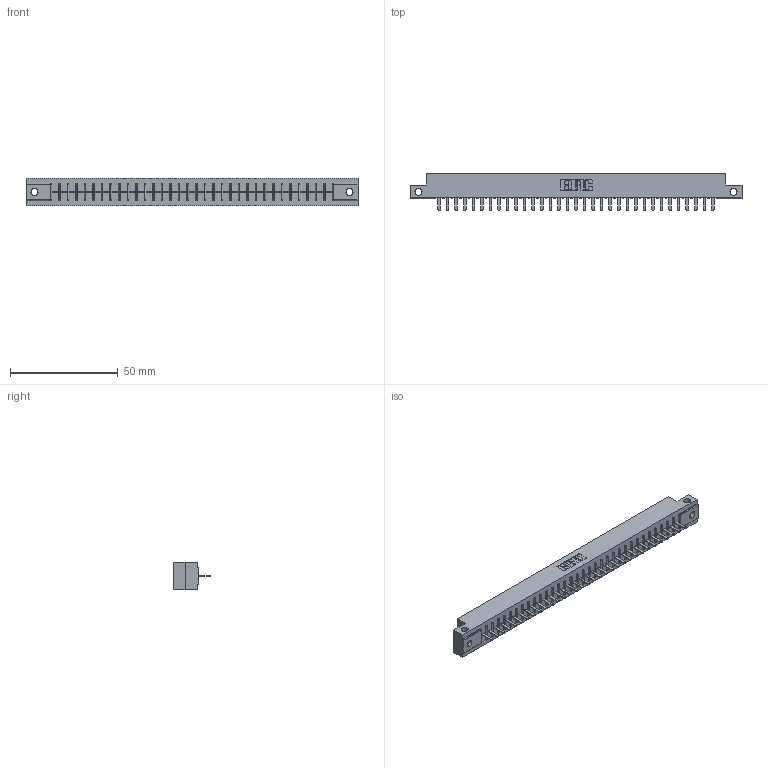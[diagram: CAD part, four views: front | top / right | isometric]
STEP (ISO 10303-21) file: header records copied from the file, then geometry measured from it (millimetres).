
FILE_DESCRIPTION (( 'STEP AP203' ), '1' );
FILE_NAME ('316-033-520-112.STEP', '2020-09-20T21:19:36', ( '' ), ( '' ), 'SwSTEP 2.0', 'SolidWorks 2020', '' );
FILE_SCHEMA (( 'CONFIG_CONTROL_DESIGN' ));
Length unit declared in the file: inch
Products named in the file (3): 306 Part_.128 Dia; 306-290-001_120; 316-033-520-112
Assembly tree (34 placements, depth 2):
  316-033-520-112
    306 Part_.128 Dia
    306-290-001_120  x33
Bounding box: 153.77 x 17.12 x 12.7 mm (x, y, z)
Volume: 16732.2 mm3; surface area: 17114.1 mm2
Topology: 34 solids, 34 shells, 2438 faces, 6853 edges, 4386 vertices
Faces by surface type: plane 1619, cylinder 687, sphere 132
Entity records: 32302 total; most frequent: CARTESIAN_POINT 5470, ORIENTED_EDGE 5378, DIRECTION 5333, EDGE_CURVE 2689, VECTOR 2083, LINE 2083, VERTEX_POINT 1698, AXIS2_PLACEMENT_3D 1625
